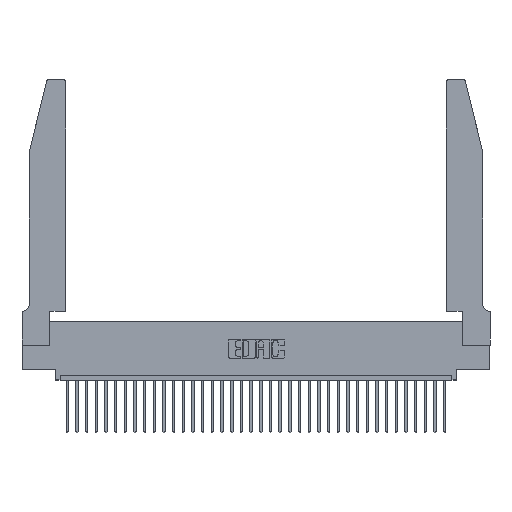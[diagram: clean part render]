
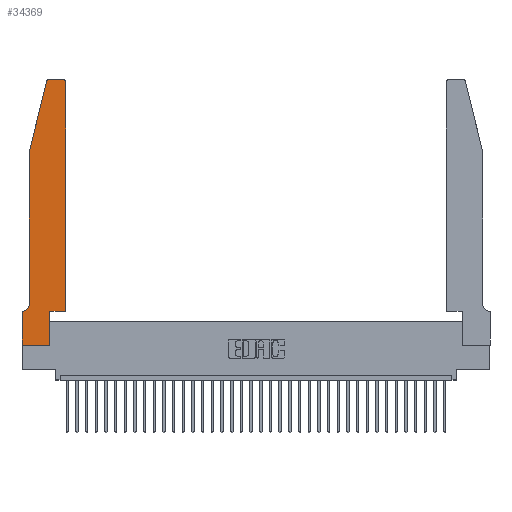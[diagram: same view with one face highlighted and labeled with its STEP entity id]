
A CAD part, top view. The second image highlights one B-rep face of the part: STEP entity #34369.
In plain terms, the highlighted planar face has unit normal (0, 0, 1).
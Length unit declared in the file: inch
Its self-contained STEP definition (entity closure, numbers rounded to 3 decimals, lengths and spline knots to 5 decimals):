
#402 = CARTESIAN_POINT ( 'NONE',  ( 0.284, 2.75, 0.37 ) ) ;
#1451 = DIRECTION ( 'NONE',  ( -1., 0., 0. ) ) ;
#1452 = DIRECTION ( 'NONE',  ( 0., 1., 0. ) ) ;
#1498 = CARTESIAN_POINT ( 'NONE',  ( 0., 0., 0.37 ) ) ;
#1800 = CARTESIAN_POINT ( 'NONE',  ( 0.0755, 2., 0.37 ) ) ;
#1935 = ORIENTED_EDGE ( 'NONE', *, *, #15119, .T. ) ;
#2452 = FACE_OUTER_BOUND ( 'NONE', #6302, .T. ) ;
#2858 = VERTEX_POINT ( 'NONE', #7778 ) ;
#2979 = VECTOR ( 'NONE', #1452, 39.37008 ) ;
#3198 = VECTOR ( 'NONE', #1451, 39.37008 ) ;
#3332 = ORIENTED_EDGE ( 'NONE', *, *, #7749, .T. ) ;
#4464 = DIRECTION ( 'NONE',  ( 1., 0., 0. ) ) ;
#4507 = DIRECTION ( 'NONE',  ( -1., 0., 0. ) ) ;
#4900 = CARTESIAN_POINT ( 'NONE',  ( 0.2605, 2.75, 0.37 ) ) ;
#4957 = CARTESIAN_POINT ( 'NONE',  ( 0.0055, 0.35, 0.37 ) ) ;
#5713 = ORIENTED_EDGE ( 'NONE', *, *, #35297, .T. ) ;
#5716 = VECTOR ( 'NONE', #19349, 39.37008 ) ;
#5730 = LINE ( 'NONE', #15247, #3198 ) ;
#5927 = DIRECTION ( 'NONE',  ( 0., 0., 1. ) ) ;
#6302 = EDGE_LOOP ( 'NONE', ( #24057, #23856, #3332, #16094, #24532, #9122, #5713, #1935, #28284, #30598, #29674, #22802 ) ) ;
#6656 = DIRECTION ( 'NONE',  ( 1., 0., 0. ) ) ;
#6997 = LINE ( 'NONE', #1800, #5716 ) ;
#7330 = DIRECTION ( 'NONE',  ( 0., 1., 0. ) ) ;
#7749 = EDGE_CURVE ( 'NONE', #18768, #26343, #6997, .T. ) ;
#7778 = CARTESIAN_POINT ( 'NONE',  ( 0.2865, 0., 0.37 ) ) ;
#8525 = DIRECTION ( 'NONE',  ( 1., 0., 0. ) ) ;
#9122 = ORIENTED_EDGE ( 'NONE', *, *, #23077, .T. ) ;
#9201 = VERTEX_POINT ( 'NONE', #21730 ) ;
#9712 = VERTEX_POINT ( 'NONE', #402 ) ;
#9787 = VECTOR ( 'NONE', #14598, 39.37008 ) ;
#9855 = CARTESIAN_POINT ( 'NONE',  ( 0.4505, 0.35, 0.37 ) ) ;
#10288 = EDGE_CURVE ( 'NONE', #15547, #31474, #28928, .T. ) ;
#10435 = CIRCLE ( 'NONE', #25199, 0.07 ) ;
#10986 = CIRCLE ( 'NONE', #34093, 0.03 ) ;
#11157 = VERTEX_POINT ( 'NONE', #13154 ) ;
#11801 = CARTESIAN_POINT ( 'NONE',  ( 0.2865, 0.35, 0.37 ) ) ;
#12708 = VECTOR ( 'NONE', #14743, 39.37008 ) ;
#12717 = VECTOR ( 'NONE', #7330, 39.37008 ) ;
#12845 = EDGE_CURVE ( 'NONE', #26343, #25367, #28975, .T. ) ;
#13154 = CARTESIAN_POINT ( 'NONE',  ( 0.4505, 2.72, 0.37 ) ) ;
#13438 = EDGE_CURVE ( 'NONE', #11157, #27444, #26838, .T. ) ;
#14180 = LINE ( 'NONE', #4900, #26908 ) ;
#14598 = DIRECTION ( 'NONE',  ( 1., 0., 0. ) ) ;
#14623 = CARTESIAN_POINT ( 'NONE',  ( 0., 0., 0.37 ) ) ;
#14671 = DIRECTION ( 'NONE',  ( 0., 0., -1. ) ) ;
#14743 = DIRECTION ( 'NONE',  ( 1., 0., 0. ) ) ;
#14776 = CARTESIAN_POINT ( 'NONE',  ( 0.284, 2.72, 0.37 ) ) ;
#14925 = CARTESIAN_POINT ( 'NONE',  ( 0.2865, 0.35, 0.37 ) ) ;
#15119 = EDGE_CURVE ( 'NONE', #25244, #2858, #15699, .T. ) ;
#15247 = CARTESIAN_POINT ( 'NONE',  ( 0.0755, 0.35, 0.37 ) ) ;
#15547 = VERTEX_POINT ( 'NONE', #11801 ) ;
#15553 = DIRECTION ( 'NONE',  ( 0., 0., 1. ) ) ;
#15699 = LINE ( 'NONE', #14623, #12708 ) ;
#15802 = LINE ( 'NONE', #14925, #2979 ) ;
#15994 = CARTESIAN_POINT ( 'NONE',  ( 0., 0., 0.37 ) ) ;
#16094 = ORIENTED_EDGE ( 'NONE', *, *, #12845, .T. ) ;
#16460 = VERTEX_POINT ( 'NONE', #4957 ) ;
#17288 = LINE ( 'NONE', #15994, #25793 ) ;
#17337 = CARTESIAN_POINT ( 'NONE',  ( 0.0755, 2., 0.37 ) ) ;
#17645 = CARTESIAN_POINT ( 'NONE',  ( 0.0055, 0.42, 0.37 ) ) ;
#18768 = VERTEX_POINT ( 'NONE', #21425 ) ;
#19349 = DIRECTION ( 'NONE',  ( -0.239, -0.971, 0. ) ) ;
#19488 = PLANE ( 'NONE',  #21249 ) ;
#19708 = EDGE_CURVE ( 'NONE', #2858, #15547, #15802, .T. ) ;
#21249 = AXIS2_PLACEMENT_3D ( 'NONE', #24803, #30293, #8525 ) ;
#21425 = CARTESIAN_POINT ( 'NONE',  ( 0.25487, 2.72718, 0.37 ) ) ;
#21432 = DIRECTION ( 'NONE',  ( -1., 0., 0. ) ) ;
#21730 = CARTESIAN_POINT ( 'NONE',  ( 0., 0.35, 0.37 ) ) ;
#21765 = CARTESIAN_POINT ( 'NONE',  ( 0.4205, 2.72, 0.37 ) ) ;
#22154 = VECTOR ( 'NONE', #24121, 39.37008 ) ;
#22346 = EDGE_CURVE ( 'NONE', #25367, #16460, #10435, .T. ) ;
#22485 = LINE ( 'NONE', #9855, #12717 ) ;
#22802 = ORIENTED_EDGE ( 'NONE', *, *, #13438, .T. ) ;
#23077 = EDGE_CURVE ( 'NONE', #16460, #9201, #5730, .T. ) ;
#23856 = ORIENTED_EDGE ( 'NONE', *, *, #29564, .T. ) ;
#24057 = ORIENTED_EDGE ( 'NONE', *, *, #26794, .T. ) ;
#24121 = DIRECTION ( 'NONE',  ( 0., -1., 0. ) ) ;
#24532 = ORIENTED_EDGE ( 'NONE', *, *, #22346, .T. ) ;
#24803 = CARTESIAN_POINT ( 'NONE',  ( 0., 0.35, 0.37 ) ) ;
#25199 = AXIS2_PLACEMENT_3D ( 'NONE', #17645, #14671, #4507 ) ;
#25211 = CARTESIAN_POINT ( 'NONE',  ( 0.0755, 0.42, 0.37 ) ) ;
#25244 = VERTEX_POINT ( 'NONE', #1498 ) ;
#25367 = VERTEX_POINT ( 'NONE', #25211 ) ;
#25793 = VECTOR ( 'NONE', #26873, 39.37008 ) ;
#26123 = CARTESIAN_POINT ( 'NONE',  ( 0.4505, 0.35, 0.37 ) ) ;
#26343 = VERTEX_POINT ( 'NONE', #17337 ) ;
#26794 = EDGE_CURVE ( 'NONE', #27444, #9712, #14180, .T. ) ;
#26838 = CIRCLE ( 'NONE', #30149, 0.03 ) ;
#26873 = DIRECTION ( 'NONE',  ( 0., -1., 0. ) ) ;
#26908 = VECTOR ( 'NONE', #21432, 39.37008 ) ;
#27443 = CARTESIAN_POINT ( 'NONE',  ( 0.4205, 2.75, 0.37 ) ) ;
#27444 = VERTEX_POINT ( 'NONE', #27443 ) ;
#27862 = CARTESIAN_POINT ( 'NONE',  ( 0.4505, 0.35, 0.37 ) ) ;
#28284 = ORIENTED_EDGE ( 'NONE', *, *, #19708, .T. ) ;
#28928 = LINE ( 'NONE', #27862, #9787 ) ;
#28975 = LINE ( 'NONE', #29358, #22154 ) ;
#29358 = CARTESIAN_POINT ( 'NONE',  ( 0.0755, 2., 0.37 ) ) ;
#29564 = EDGE_CURVE ( 'NONE', #9712, #18768, #10986, .T. ) ;
#29674 = ORIENTED_EDGE ( 'NONE', *, *, #29678, .T. ) ;
#29678 = EDGE_CURVE ( 'NONE', #31474, #11157, #22485, .T. ) ;
#30149 = AXIS2_PLACEMENT_3D ( 'NONE', #21765, #5927, #6656 ) ;
#30293 = DIRECTION ( 'NONE',  ( 0., 0., 1. ) ) ;
#30598 = ORIENTED_EDGE ( 'NONE', *, *, #10288, .T. ) ;
#31474 = VERTEX_POINT ( 'NONE', #26123 ) ;
#34093 = AXIS2_PLACEMENT_3D ( 'NONE', #14776, #15553, #4464 ) ;
#34369 = ADVANCED_FACE ( 'NONE', ( #2452 ), #19488, .T. ) ;
#35297 = EDGE_CURVE ( 'NONE', #9201, #25244, #17288, .T. ) ;
